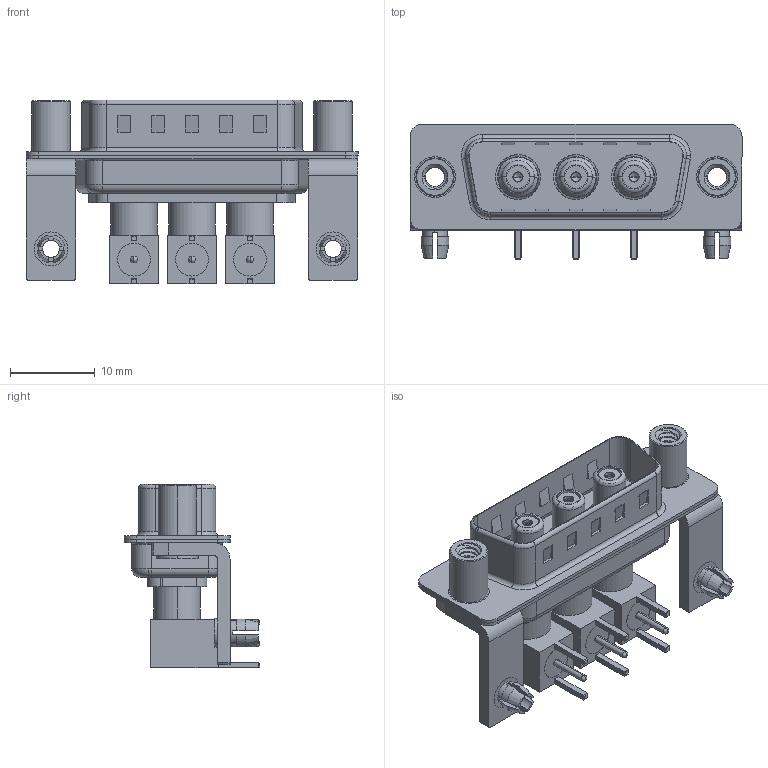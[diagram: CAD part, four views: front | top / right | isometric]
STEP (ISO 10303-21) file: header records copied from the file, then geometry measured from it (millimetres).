
FILE_DESCRIPTION (( 'STEP AP203' ), '1' );
FILE_NAME ('629-3W3-240-5N5.STEP', '2022-05-05T02:13:41', ( '' ), ( '' ), 'SwSTEP 2.0', 'SolidWorks 2020', '' );
FILE_SCHEMA (( 'CONFIG_CONTROL_DESIGN' ));
Length unit declared in the file: millimetre
Products named in the file (17): Locking Collar; Co-Ax Jack Assy_RA; Insulator Socket; 629Combo Shell Rear_15 Contacts; 629Combo Housing_3W3; 629Combo Stabilizer Bracket; 629-3W3-240-5N5; Insulator Socket 2; 629Combo Threaded Standoff_5; 629Combo Shell Front_15 Contacts; RA Back Shell; 629Combo Board Lock; Socket_RA; Insulator RA Pin; Co-Ax Jack_RA PC Tail
Assembly tree (33 placements, depth 3):
  629-3W3-240-5N5
    629Combo Housing_3W3
    629Combo Shell Rear_15 Contacts
    629Combo Shell Front_15 Contacts
    629Combo Stabilizer Bracket  x2
    629Combo Board Lock  x2
    629Combo Threaded Standoff_5  x2
    Co-Ax Jack Assy_RA
      Co-Ax Jack_RA PC Tail
      Insulator Socket
      Insulator Socket 2
      Locking Collar
      Socket_RA
      RA Back Shell
      Insulator RA Pin
    Co-Ax Jack Assy_RA
      Co-Ax Jack_RA PC Tail
      Insulator Socket
      Insulator Socket 2
      Locking Collar
      Socket_RA
      RA Back Shell
      Insulator RA Pin
    Co-Ax Jack Assy_RA
      Co-Ax Jack_RA PC Tail
      Insulator Socket
      Insulator Socket 2
      Locking Collar
      Socket_RA
      RA Back Shell
      Insulator RA Pin
Bounding box: 39.2 x 16 x 21.71 mm (x, y, z)
Volume: 3129.6 mm3; surface area: 8648 mm2
Topology: 30 solids, 30 shells, 976 faces, 2376 edges, 1495 vertices
Faces by surface type: cylinder 426, plane 380, cone 87, torus 68, bspline 9, sphere 6
Entity records: 20897 total; most frequent: CARTESIAN_POINT 5024, DIRECTION 2999, ORIENTED_EDGE 2750, EDGE_CURVE 1375, AXIS2_PLACEMENT_3D 1135, VERTEX_POINT 872, VECTOR 729, LINE 729
